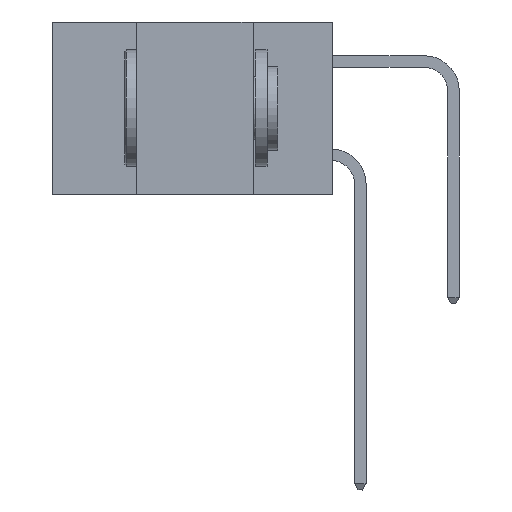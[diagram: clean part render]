
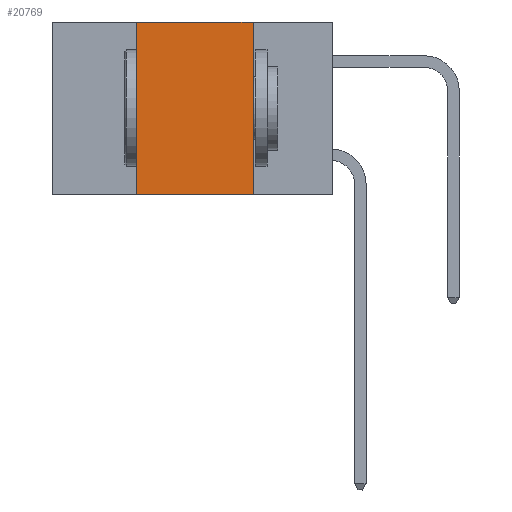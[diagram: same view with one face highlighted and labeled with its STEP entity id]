
A CAD part, left-side view. The second image highlights one B-rep face of the part: STEP entity #20769.
In plain terms, the highlighted planar face has unit normal (-1, 0, 0).
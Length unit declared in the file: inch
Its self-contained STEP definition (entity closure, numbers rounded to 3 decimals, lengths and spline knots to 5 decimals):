
#126 = PLANE ( 'NONE',  #14420 ) ;
#933 = CARTESIAN_POINT ( 'NONE',  ( 0., 0.42, -0.37 ) ) ;
#940 = VECTOR ( 'NONE', #1656, 39.37008 ) ;
#1656 = DIRECTION ( 'NONE',  ( 0., -1., 0. ) ) ;
#2589 = CARTESIAN_POINT ( 'NONE',  ( 0., 0.42, 0. ) ) ;
#3422 = VECTOR ( 'NONE', #10903, 39.37008 ) ;
#3892 = EDGE_CURVE ( 'NONE', #4995, #18903, #18658, .T. ) ;
#4421 = FACE_OUTER_BOUND ( 'NONE', #5602, .T. ) ;
#4995 = VERTEX_POINT ( 'NONE', #21130 ) ;
#5196 = LINE ( 'NONE', #24674, #6339 ) ;
#5510 = EDGE_CURVE ( 'NONE', #18490, #7410, #15316, .T. ) ;
#5602 = EDGE_LOOP ( 'NONE', ( #10460, #20098, #17607, #24821 ) ) ;
#5997 = EDGE_CURVE ( 'NONE', #18903, #18490, #5196, .T. ) ;
#6084 = CARTESIAN_POINT ( 'NONE',  ( 0., 0.17, -0.37 ) ) ;
#6339 = VECTOR ( 'NONE', #20816, 39.37008 ) ;
#7410 = VERTEX_POINT ( 'NONE', #6084 ) ;
#10460 = ORIENTED_EDGE ( 'NONE', *, *, #5510, .F. ) ;
#10834 = EDGE_CURVE ( 'NONE', #4995, #7410, #17818, .T. ) ;
#10903 = DIRECTION ( 'NONE',  ( 0., 0., 1. ) ) ;
#11739 = CARTESIAN_POINT ( 'NONE',  ( 0., 0.6, -0.37 ) ) ;
#12166 = CARTESIAN_POINT ( 'NONE',  ( 0., 0.6, 0. ) ) ;
#13720 = DIRECTION ( 'NONE',  ( 0., 0., -1. ) ) ;
#14420 = AXIS2_PLACEMENT_3D ( 'NONE', #12166, #23526, #13720 ) ;
#15316 = LINE ( 'NONE', #24830, #20346 ) ;
#17607 = ORIENTED_EDGE ( 'NONE', *, *, #3892, .F. ) ;
#17818 = LINE ( 'NONE', #11739, #940 ) ;
#18490 = VERTEX_POINT ( 'NONE', #22159 ) ;
#18658 = LINE ( 'NONE', #933, #3422 ) ;
#18903 = VERTEX_POINT ( 'NONE', #2589 ) ;
#20098 = ORIENTED_EDGE ( 'NONE', *, *, #5997, .F. ) ;
#20346 = VECTOR ( 'NONE', #23166, 39.37008 ) ;
#20769 = ADVANCED_FACE ( 'NONE', ( #4421 ), #126, .F. ) ;
#20816 = DIRECTION ( 'NONE',  ( 0., -1., 0. ) ) ;
#21130 = CARTESIAN_POINT ( 'NONE',  ( 0., 0.42, -0.37 ) ) ;
#22159 = CARTESIAN_POINT ( 'NONE',  ( 0., 0.17, 0. ) ) ;
#23166 = DIRECTION ( 'NONE',  ( 0., 0., -1. ) ) ;
#23526 = DIRECTION ( 'NONE',  ( 1., 0., 0. ) ) ;
#24674 = CARTESIAN_POINT ( 'NONE',  ( 0., 0.6, 0. ) ) ;
#24821 = ORIENTED_EDGE ( 'NONE', *, *, #10834, .T. ) ;
#24830 = CARTESIAN_POINT ( 'NONE',  ( 0., 0.17, -0.37 ) ) ;
